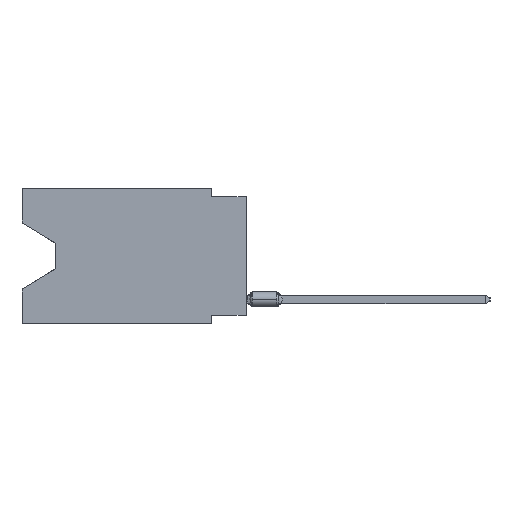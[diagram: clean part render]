
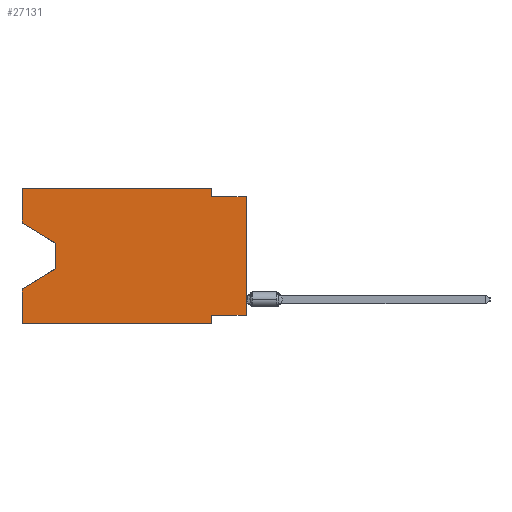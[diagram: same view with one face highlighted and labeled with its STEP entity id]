
A CAD part, left-side view. The second image highlights one B-rep face of the part: STEP entity #27131.
In plain terms, the highlighted planar face has unit normal (-1, 0, 0).
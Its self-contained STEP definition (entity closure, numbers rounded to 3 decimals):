
#111 = CARTESIAN_POINT ( 'NONE',  ( 0., 16.383, -9.906 ) ) ;
#722 = EDGE_CURVE ( 'NONE', #6269, #4360, #25655, .T. ) ;
#902 = DIRECTION ( 'NONE',  ( 0., 0., 1. ) ) ;
#1264 = ORIENTED_EDGE ( 'NONE', *, *, #9632, .T. ) ;
#1313 = VECTOR ( 'NONE', #11024, 1000. ) ;
#2627 = VERTEX_POINT ( 'NONE', #20238 ) ;
#2647 = EDGE_CURVE ( 'NONE', #27434, #7149, #9375, .T. ) ;
#3580 = LINE ( 'NONE', #19732, #30935 ) ;
#3806 = ORIENTED_EDGE ( 'NONE', *, *, #25818, .T. ) ;
#4360 = VERTEX_POINT ( 'NONE', #28044 ) ;
#4553 = AXIS2_PLACEMENT_3D ( 'NONE', #17811, #15177, #14645 ) ;
#4659 = LINE ( 'NONE', #15390, #28429 ) ;
#4683 = VECTOR ( 'NONE', #30760, 1000. ) ;
#6269 = VERTEX_POINT ( 'NONE', #19941 ) ;
#7101 = FACE_OUTER_BOUND ( 'NONE', #29208, .T. ) ;
#7149 = VERTEX_POINT ( 'NONE', #11010 ) ;
#7712 = CARTESIAN_POINT ( 'NONE',  ( 0., 16.383, -2.546 ) ) ;
#7995 = DIRECTION ( 'NONE',  ( 0., -1., 0. ) ) ;
#8315 = VECTOR ( 'NONE', #14769, 1000. ) ;
#8567 = EDGE_CURVE ( 'NONE', #32053, #15458, #17199, .T. ) ;
#8879 = EDGE_CURVE ( 'NONE', #24991, #2627, #4659, .T. ) ;
#8944 = CARTESIAN_POINT ( 'NONE',  ( 0., 16.383, -7.36 ) ) ;
#9074 = CARTESIAN_POINT ( 'NONE',  ( 0., 0., -0.635 ) ) ;
#9375 = LINE ( 'NONE', #17264, #4683 ) ;
#9632 = EDGE_CURVE ( 'NONE', #6269, #27434, #31747, .T. ) ;
#11010 = CARTESIAN_POINT ( 'NONE',  ( 0., 13.97, -5.893 ) ) ;
#11024 = DIRECTION ( 'NONE',  ( 0., 0., -1. ) ) ;
#11083 = CARTESIAN_POINT ( 'NONE',  ( 0., 2.54, -9.906 ) ) ;
#11094 = EDGE_CURVE ( 'NONE', #32053, #31736, #20347, .T. ) ;
#11314 = ORIENTED_EDGE ( 'NONE', *, *, #32464, .F. ) ;
#11629 = CARTESIAN_POINT ( 'NONE',  ( 0., 0., 0. ) ) ;
#11864 = DIRECTION ( 'NONE',  ( 0., 1., 0. ) ) ;
#12382 = ORIENTED_EDGE ( 'NONE', *, *, #29478, .F. ) ;
#14645 = DIRECTION ( 'NONE',  ( 0., 0., -1. ) ) ;
#14769 = DIRECTION ( 'NONE',  ( 0., -0.855, -0.519 ) ) ;
#15177 = DIRECTION ( 'NONE',  ( 1., 0., 0. ) ) ;
#15248 = VECTOR ( 'NONE', #15757, 1000. ) ;
#15390 = CARTESIAN_POINT ( 'NONE',  ( 0., 2.54, 0. ) ) ;
#15458 = VERTEX_POINT ( 'NONE', #11083 ) ;
#15757 = DIRECTION ( 'NONE',  ( 0., -1., 0. ) ) ;
#15860 = EDGE_CURVE ( 'NONE', #31750, #27286, #22235, .T. ) ;
#16367 = VECTOR ( 'NONE', #17405, 1000. ) ;
#17199 = LINE ( 'NONE', #24379, #21152 ) ;
#17264 = CARTESIAN_POINT ( 'NONE',  ( 0., 13.97, -4.013 ) ) ;
#17405 = DIRECTION ( 'NONE',  ( 0., 0., 1. ) ) ;
#17811 = CARTESIAN_POINT ( 'NONE',  ( 0., 16.383, 0. ) ) ;
#17930 = ORIENTED_EDGE ( 'NONE', *, *, #8567, .T. ) ;
#18289 = VECTOR ( 'NONE', #7995, 1000. ) ;
#19252 = EDGE_CURVE ( 'NONE', #2627, #32209, #32221, .T. ) ;
#19279 = LINE ( 'NONE', #29793, #1313 ) ;
#19647 = DIRECTION ( 'NONE',  ( 0., -1., 0. ) ) ;
#19702 = LINE ( 'NONE', #11629, #26951 ) ;
#19732 = CARTESIAN_POINT ( 'NONE',  ( 0., 13.97, -5.893 ) ) ;
#19941 = CARTESIAN_POINT ( 'NONE',  ( 0., 16.383, -2.546 ) ) ;
#20238 = CARTESIAN_POINT ( 'NONE',  ( 0., 2.54, -0.635 ) ) ;
#20347 = LINE ( 'NONE', #34198, #30844 ) ;
#20435 = PLANE ( 'NONE',  #4553 ) ;
#20446 = CARTESIAN_POINT ( 'NONE',  ( 0., 2.54, 0. ) ) ;
#21152 = VECTOR ( 'NONE', #19647, 1000. ) ;
#22235 = LINE ( 'NONE', #24676, #33930 ) ;
#22287 = ORIENTED_EDGE ( 'NONE', *, *, #722, .F. ) ;
#22630 = CARTESIAN_POINT ( 'NONE',  ( 0., 0., -9.271 ) ) ;
#22848 = CARTESIAN_POINT ( 'NONE',  ( 0., 16.383, 0. ) ) ;
#23582 = CARTESIAN_POINT ( 'NONE',  ( 0., 2.54, -9.271 ) ) ;
#23987 = CARTESIAN_POINT ( 'NONE',  ( 0., 0., -0.635 ) ) ;
#24379 = CARTESIAN_POINT ( 'NONE',  ( 0., 16.383, -9.906 ) ) ;
#24676 = CARTESIAN_POINT ( 'NONE',  ( 0., 0., -9.271 ) ) ;
#24991 = VERTEX_POINT ( 'NONE', #20446 ) ;
#25193 = EDGE_CURVE ( 'NONE', #31750, #32209, #19702, .T. ) ;
#25655 = LINE ( 'NONE', #22848, #16367 ) ;
#25818 = EDGE_CURVE ( 'NONE', #7149, #31736, #3580, .T. ) ;
#26083 = DIRECTION ( 'NONE',  ( 0., 0., -1. ) ) ;
#26951 = VECTOR ( 'NONE', #902, 1000. ) ;
#27131 = ADVANCED_FACE ( 'NONE', ( #7101 ), #20435, .F. ) ;
#27286 = VERTEX_POINT ( 'NONE', #23582 ) ;
#27434 = VERTEX_POINT ( 'NONE', #32170 ) ;
#27628 = DIRECTION ( 'NONE',  ( 0., 0.855, -0.519 ) ) ;
#27973 = ORIENTED_EDGE ( 'NONE', *, *, #2647, .T. ) ;
#28044 = CARTESIAN_POINT ( 'NONE',  ( 0., 16.383, 0. ) ) ;
#28090 = ORIENTED_EDGE ( 'NONE', *, *, #19252, .F. ) ;
#28429 = VECTOR ( 'NONE', #26083, 1000. ) ;
#29208 = EDGE_LOOP ( 'NONE', ( #1264, #27973, #3806, #31508, #17930, #12382, #30938, #32396, #28090, #30314, #11314, #22287 ) ) ;
#29478 = EDGE_CURVE ( 'NONE', #27286, #15458, #19279, .T. ) ;
#29793 = CARTESIAN_POINT ( 'NONE',  ( 0., 2.54, -9.906 ) ) ;
#30314 = ORIENTED_EDGE ( 'NONE', *, *, #8879, .F. ) ;
#30760 = DIRECTION ( 'NONE',  ( 0., 0., -1. ) ) ;
#30844 = VECTOR ( 'NONE', #31221, 1000. ) ;
#30935 = VECTOR ( 'NONE', #27628, 1000. ) ;
#30938 = ORIENTED_EDGE ( 'NONE', *, *, #15860, .F. ) ;
#31221 = DIRECTION ( 'NONE',  ( 0., 0., 1. ) ) ;
#31508 = ORIENTED_EDGE ( 'NONE', *, *, #11094, .F. ) ;
#31736 = VERTEX_POINT ( 'NONE', #8944 ) ;
#31747 = LINE ( 'NONE', #7712, #8315 ) ;
#31750 = VERTEX_POINT ( 'NONE', #22630 ) ;
#32053 = VERTEX_POINT ( 'NONE', #111 ) ;
#32170 = CARTESIAN_POINT ( 'NONE',  ( 0., 13.97, -4.013 ) ) ;
#32209 = VERTEX_POINT ( 'NONE', #9074 ) ;
#32221 = LINE ( 'NONE', #23987, #15248 ) ;
#32366 = LINE ( 'NONE', #34504, #18289 ) ;
#32396 = ORIENTED_EDGE ( 'NONE', *, *, #25193, .T. ) ;
#32464 = EDGE_CURVE ( 'NONE', #4360, #24991, #32366, .T. ) ;
#33930 = VECTOR ( 'NONE', #11864, 1000. ) ;
#34198 = CARTESIAN_POINT ( 'NONE',  ( 0., 16.383, 0. ) ) ;
#34504 = CARTESIAN_POINT ( 'NONE',  ( 0., 16.383, 0. ) ) ;
